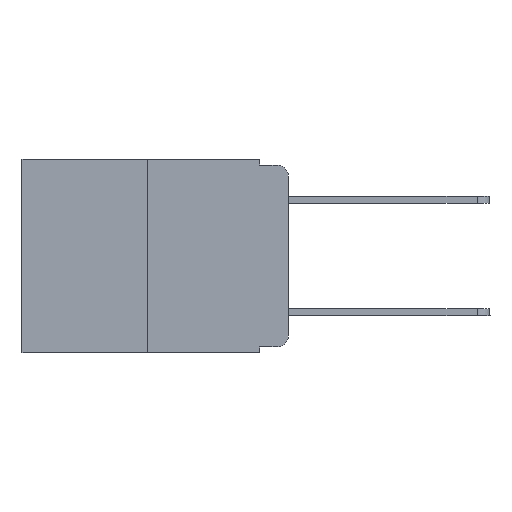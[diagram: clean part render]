
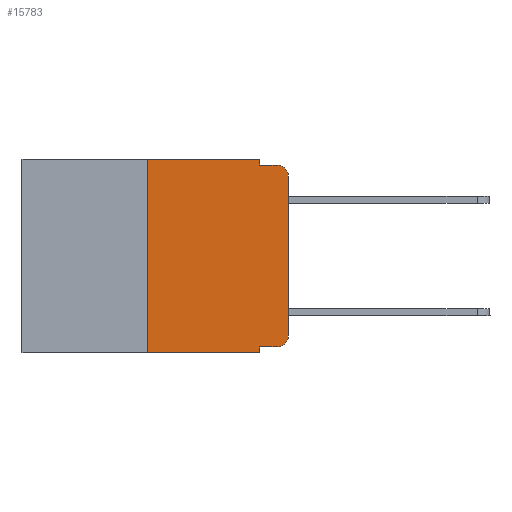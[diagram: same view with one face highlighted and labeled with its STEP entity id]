
A CAD part, left-side view. The second image highlights one B-rep face of the part: STEP entity #15783.
In plain terms, the highlighted planar face has unit normal (-1, 0, 0).
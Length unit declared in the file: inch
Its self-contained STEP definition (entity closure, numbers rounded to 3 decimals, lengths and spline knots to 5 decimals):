
#187 = AXIS2_PLACEMENT_3D ( 'NONE', #12394, #19568, #8143 ) ;
#333 = EDGE_CURVE ( 'NONE', #11158, #900, #6692, .T. ) ;
#861 = CARTESIAN_POINT ( 'NONE',  ( 0., 0.051, 0. ) ) ;
#900 = VERTEX_POINT ( 'NONE', #1061 ) ;
#1061 = CARTESIAN_POINT ( 'NONE',  ( 0., 0.051, -0.01 ) ) ;
#2867 = CARTESIAN_POINT ( 'NONE',  ( 0., 0.02, -0.03 ) ) ;
#3086 = VERTEX_POINT ( 'NONE', #19464 ) ;
#3567 = EDGE_CURVE ( 'NONE', #7036, #22924, #11654, .T. ) ;
#3705 = CARTESIAN_POINT ( 'NONE',  ( 0., 0.473, 0. ) ) ;
#3844 = VERTEX_POINT ( 'NONE', #10560 ) ;
#4123 = EDGE_CURVE ( 'NONE', #22924, #8742, #8536, .T. ) ;
#4654 = EDGE_CURVE ( 'NONE', #8397, #3844, #21094, .T. ) ;
#4729 = CARTESIAN_POINT ( 'NONE',  ( 0., 0.051, -0.01 ) ) ;
#6186 = DIRECTION ( 'NONE',  ( 0., -1., 0. ) ) ;
#6377 = CARTESIAN_POINT ( 'NONE',  ( 0., 0.02, -0.333 ) ) ;
#6599 = DIRECTION ( 'NONE',  ( 0., 0., -1. ) ) ;
#6692 = LINE ( 'NONE', #861, #14910 ) ;
#6705 = ORIENTED_EDGE ( 'NONE', *, *, #3567, .T. ) ;
#6753 = CARTESIAN_POINT ( 'NONE',  ( 0., 0.25, 0. ) ) ;
#7036 = VERTEX_POINT ( 'NONE', #16480 ) ;
#7255 = VECTOR ( 'NONE', #6599, 39.37008 ) ;
#7362 = PLANE ( 'NONE',  #9226 ) ;
#7593 = CARTESIAN_POINT ( 'NONE',  ( 0., 0.25, 0. ) ) ;
#8104 = LINE ( 'NONE', #18970, #21287 ) ;
#8143 = DIRECTION ( 'NONE',  ( 0., 0., -1. ) ) ;
#8386 = LINE ( 'NONE', #22816, #20908 ) ;
#8397 = VERTEX_POINT ( 'NONE', #9390 ) ;
#8536 = CIRCLE ( 'NONE', #187, 0.02 ) ;
#8568 = ORIENTED_EDGE ( 'NONE', *, *, #21658, .F. ) ;
#8742 = VERTEX_POINT ( 'NONE', #19866 ) ;
#9226 = AXIS2_PLACEMENT_3D ( 'NONE', #17956, #19757, #14389 ) ;
#9323 = ORIENTED_EDGE ( 'NONE', *, *, #16323, .F. ) ;
#9390 = CARTESIAN_POINT ( 'NONE',  ( 0., 0., -0.03 ) ) ;
#9673 = DIRECTION ( 'NONE',  ( 0., 0., 1. ) ) ;
#9913 = EDGE_CURVE ( 'NONE', #900, #3844, #12000, .T. ) ;
#10300 = ORIENTED_EDGE ( 'NONE', *, *, #9913, .F. ) ;
#10560 = CARTESIAN_POINT ( 'NONE',  ( 0., 0.02, -0.01 ) ) ;
#10862 = ORIENTED_EDGE ( 'NONE', *, *, #16561, .T. ) ;
#10945 = FACE_OUTER_BOUND ( 'NONE', #15080, .T. ) ;
#11158 = VERTEX_POINT ( 'NONE', #19170 ) ;
#11654 = LINE ( 'NONE', #22373, #18811 ) ;
#11840 = LINE ( 'NONE', #21014, #7255 ) ;
#12000 = LINE ( 'NONE', #4729, #20483 ) ;
#12335 = ORIENTED_EDGE ( 'NONE', *, *, #333, .F. ) ;
#12394 = CARTESIAN_POINT ( 'NONE',  ( 0., 0.02, -0.313 ) ) ;
#13614 = DIRECTION ( 'NONE',  ( 0., 0., -1. ) ) ;
#14389 = DIRECTION ( 'NONE',  ( 0., 0., -1. ) ) ;
#14539 = DIRECTION ( 'NONE',  ( 0., -1., 0. ) ) ;
#14822 = VERTEX_POINT ( 'NONE', #15673 ) ;
#14850 = DIRECTION ( 'NONE',  ( 0., 0., 1. ) ) ;
#14910 = VECTOR ( 'NONE', #13614, 39.37008 ) ;
#15080 = EDGE_LOOP ( 'NONE', ( #16709, #20019, #10300, #12335, #17525, #9323, #10862, #8568, #6705, #16529 ) ) ;
#15673 = CARTESIAN_POINT ( 'NONE',  ( 0., 0.25, -0.343 ) ) ;
#15783 = ADVANCED_FACE ( 'NONE', ( #10945 ), #7362, .F. ) ;
#15808 = LINE ( 'NONE', #6753, #21423 ) ;
#15941 = DIRECTION ( 'NONE',  ( 0., 0., -1. ) ) ;
#16323 = EDGE_CURVE ( 'NONE', #14822, #19265, #15808, .T. ) ;
#16480 = CARTESIAN_POINT ( 'NONE',  ( 0., 0.051, -0.333 ) ) ;
#16529 = ORIENTED_EDGE ( 'NONE', *, *, #4123, .T. ) ;
#16561 = EDGE_CURVE ( 'NONE', #14822, #3086, #8386, .T. ) ;
#16709 = ORIENTED_EDGE ( 'NONE', *, *, #18579, .T. ) ;
#17477 = DIRECTION ( 'NONE',  ( 0., -1., 0. ) ) ;
#17525 = ORIENTED_EDGE ( 'NONE', *, *, #18888, .F. ) ;
#17956 = CARTESIAN_POINT ( 'NONE',  ( 0., 0.473, 0. ) ) ;
#18579 = EDGE_CURVE ( 'NONE', #8742, #8397, #8104, .T. ) ;
#18811 = VECTOR ( 'NONE', #6186, 39.37008 ) ;
#18880 = AXIS2_PLACEMENT_3D ( 'NONE', #2867, #23098, #15941 ) ;
#18888 = EDGE_CURVE ( 'NONE', #19265, #11158, #20265, .T. ) ;
#18970 = CARTESIAN_POINT ( 'NONE',  ( 0., 0., 0. ) ) ;
#19170 = CARTESIAN_POINT ( 'NONE',  ( 0., 0.051, 0. ) ) ;
#19265 = VERTEX_POINT ( 'NONE', #7593 ) ;
#19386 = VECTOR ( 'NONE', #14539, 39.37008 ) ;
#19464 = CARTESIAN_POINT ( 'NONE',  ( 0., 0.051, -0.343 ) ) ;
#19568 = DIRECTION ( 'NONE',  ( -1., 0., 0. ) ) ;
#19757 = DIRECTION ( 'NONE',  ( 1., 0., 0. ) ) ;
#19866 = CARTESIAN_POINT ( 'NONE',  ( 0., 0., -0.313 ) ) ;
#20019 = ORIENTED_EDGE ( 'NONE', *, *, #4654, .T. ) ;
#20265 = LINE ( 'NONE', #3705, #19386 ) ;
#20483 = VECTOR ( 'NONE', #17477, 39.37008 ) ;
#20908 = VECTOR ( 'NONE', #20922, 39.37008 ) ;
#20922 = DIRECTION ( 'NONE',  ( 0., -1., 0. ) ) ;
#21014 = CARTESIAN_POINT ( 'NONE',  ( 0., 0.051, 0. ) ) ;
#21094 = CIRCLE ( 'NONE', #18880, 0.02 ) ;
#21287 = VECTOR ( 'NONE', #9673, 39.37008 ) ;
#21423 = VECTOR ( 'NONE', #14850, 39.37008 ) ;
#21658 = EDGE_CURVE ( 'NONE', #7036, #3086, #11840, .T. ) ;
#22373 = CARTESIAN_POINT ( 'NONE',  ( 0., 0.051, -0.333 ) ) ;
#22816 = CARTESIAN_POINT ( 'NONE',  ( 0., 0.473, -0.343 ) ) ;
#22924 = VERTEX_POINT ( 'NONE', #6377 ) ;
#23098 = DIRECTION ( 'NONE',  ( -1., 0., 0. ) ) ;
